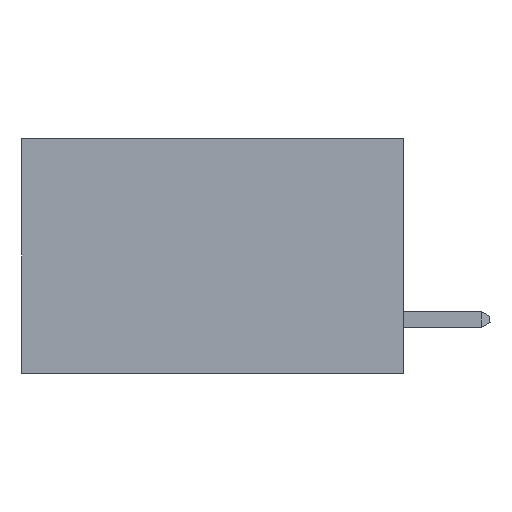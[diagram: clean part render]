
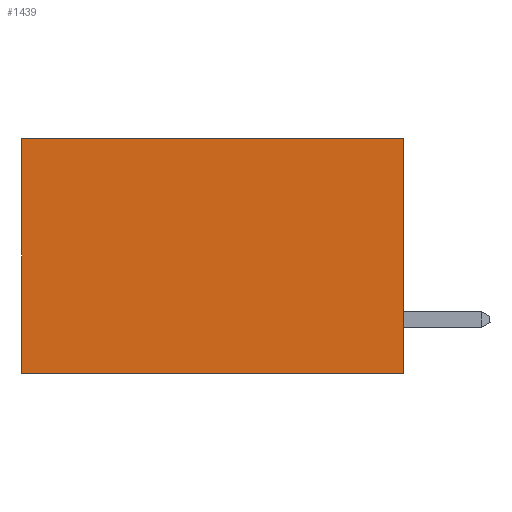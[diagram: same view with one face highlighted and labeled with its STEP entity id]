
A CAD part, left-side view. The second image highlights one B-rep face of the part: STEP entity #1439.
In plain terms, the highlighted planar face has unit normal (-1, 0, 0).
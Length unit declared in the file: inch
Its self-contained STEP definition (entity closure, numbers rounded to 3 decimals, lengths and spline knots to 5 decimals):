
#168 = EDGE_LOOP ( 'NONE', ( #11312, #12499, #3975, #6919 ) ) ;
#1439 = ADVANCED_FACE ( 'NONE', ( #4908 ), #8639, .F. ) ;
#2033 = LINE ( 'NONE', #4573, #11025 ) ;
#2555 = DIRECTION ( 'NONE',  ( 0., 0., -1. ) ) ;
#3975 = ORIENTED_EDGE ( 'NONE', *, *, #10807, .F. ) ;
#4197 = EDGE_CURVE ( 'NONE', #13788, #8007, #5165, .T. ) ;
#4289 = AXIS2_PLACEMENT_3D ( 'NONE', #12025, #6064, #2555 ) ;
#4347 = CARTESIAN_POINT ( 'NONE',  ( 0.2875, 0., -0.37 ) ) ;
#4573 = CARTESIAN_POINT ( 'NONE',  ( 0.2875, 0., 0. ) ) ;
#4861 = DIRECTION ( 'NONE',  ( 0., 0., -1. ) ) ;
#4908 = FACE_OUTER_BOUND ( 'NONE', #168, .T. ) ;
#5165 = LINE ( 'NONE', #6148, #15136 ) ;
#6064 = DIRECTION ( 'NONE',  ( 1., 0., 0. ) ) ;
#6148 = CARTESIAN_POINT ( 'NONE',  ( 0.2875, 0.6, 0. ) ) ;
#6779 = CARTESIAN_POINT ( 'NONE',  ( 0.2875, 0., 0. ) ) ;
#6919 = ORIENTED_EDGE ( 'NONE', *, *, #14913, .T. ) ;
#6986 = LINE ( 'NONE', #7857, #8288 ) ;
#7857 = CARTESIAN_POINT ( 'NONE',  ( 0.2875, 0., -0.37 ) ) ;
#8007 = VERTEX_POINT ( 'NONE', #12245 ) ;
#8288 = VECTOR ( 'NONE', #15037, 39.37008 ) ;
#8310 = CARTESIAN_POINT ( 'NONE',  ( 0.2875, 0.6, 0. ) ) ;
#8639 = PLANE ( 'NONE',  #4289 ) ;
#8782 = VECTOR ( 'NONE', #4861, 39.37008 ) ;
#9295 = DIRECTION ( 'NONE',  ( 0., 1., 0. ) ) ;
#9791 = VERTEX_POINT ( 'NONE', #6779 ) ;
#10807 = EDGE_CURVE ( 'NONE', #9791, #11780, #14469, .T. ) ;
#11025 = VECTOR ( 'NONE', #9295, 39.37008 ) ;
#11312 = ORIENTED_EDGE ( 'NONE', *, *, #4197, .T. ) ;
#11780 = VERTEX_POINT ( 'NONE', #4347 ) ;
#12025 = CARTESIAN_POINT ( 'NONE',  ( 0.2875, 0., 0. ) ) ;
#12195 = CARTESIAN_POINT ( 'NONE',  ( 0.2875, 0., 0. ) ) ;
#12245 = CARTESIAN_POINT ( 'NONE',  ( 0.2875, 0.6, -0.37 ) ) ;
#12499 = ORIENTED_EDGE ( 'NONE', *, *, #15146, .F. ) ;
#13788 = VERTEX_POINT ( 'NONE', #8310 ) ;
#14169 = DIRECTION ( 'NONE',  ( 0., 0., -1. ) ) ;
#14469 = LINE ( 'NONE', #12195, #8782 ) ;
#14913 = EDGE_CURVE ( 'NONE', #9791, #13788, #2033, .T. ) ;
#15037 = DIRECTION ( 'NONE',  ( 0., 1., 0. ) ) ;
#15136 = VECTOR ( 'NONE', #14169, 39.37008 ) ;
#15146 = EDGE_CURVE ( 'NONE', #11780, #8007, #6986, .T. ) ;
